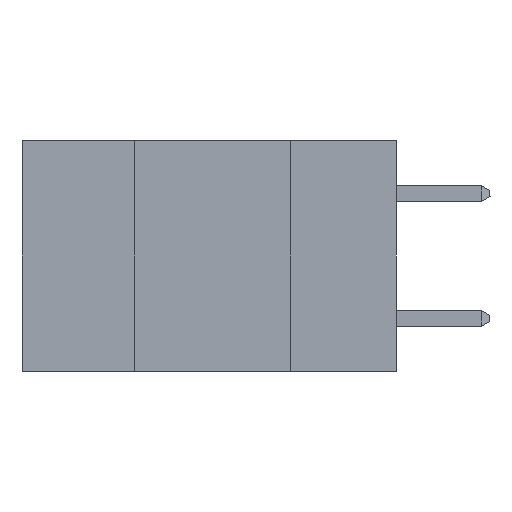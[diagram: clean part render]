
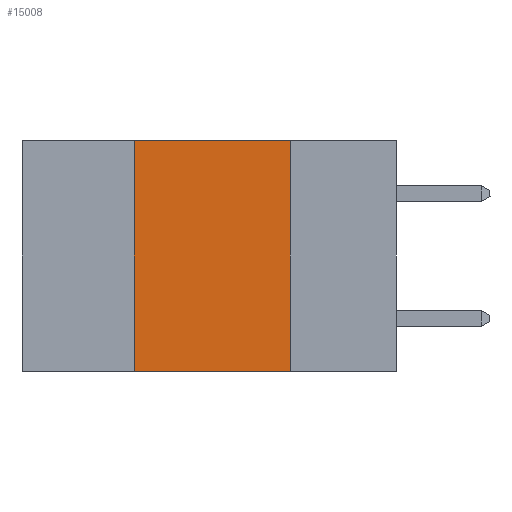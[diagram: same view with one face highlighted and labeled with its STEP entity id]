
A CAD part, left-side view. The second image highlights one B-rep face of the part: STEP entity #15008.
In plain terms, the highlighted planar face has unit normal (-1, 0, 0).
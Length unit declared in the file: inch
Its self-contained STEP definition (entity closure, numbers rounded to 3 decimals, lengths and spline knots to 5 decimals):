
#212 = EDGE_CURVE ( 'NONE', #6444, #10614, #8181, .T. ) ;
#1032 = FACE_OUTER_BOUND ( 'NONE', #9208, .T. ) ;
#1127 = CARTESIAN_POINT ( 'NONE',  ( 0., 0.42, 0. ) ) ;
#1214 = LINE ( 'NONE', #11741, #7696 ) ;
#1249 = VECTOR ( 'NONE', #15882, 39.37008 ) ;
#1621 = CARTESIAN_POINT ( 'NONE',  ( 0., 0.42, 0. ) ) ;
#1800 = VECTOR ( 'NONE', #9566, 39.37008 ) ;
#2646 = DIRECTION ( 'NONE',  ( 1., 0., 0. ) ) ;
#3077 = EDGE_CURVE ( 'NONE', #6444, #17207, #4253, .T. ) ;
#4253 = LINE ( 'NONE', #5194, #1800 ) ;
#4759 = CARTESIAN_POINT ( 'NONE',  ( 0., 0.17, 0. ) ) ;
#5026 = ORIENTED_EDGE ( 'NONE', *, *, #17885, .F. ) ;
#5194 = CARTESIAN_POINT ( 'NONE',  ( 0., 0.6, -0.37 ) ) ;
#5376 = ORIENTED_EDGE ( 'NONE', *, *, #6539, .F. ) ;
#6444 = VERTEX_POINT ( 'NONE', #7243 ) ;
#6539 = EDGE_CURVE ( 'NONE', #14490, #17207, #9212, .T. ) ;
#7243 = CARTESIAN_POINT ( 'NONE',  ( 0., 0.42, -0.37 ) ) ;
#7254 = DIRECTION ( 'NONE',  ( 0., -1., 0. ) ) ;
#7696 = VECTOR ( 'NONE', #7254, 39.37008 ) ;
#8181 = LINE ( 'NONE', #1621, #1249 ) ;
#8528 = VECTOR ( 'NONE', #16338, 39.37008 ) ;
#8595 = PLANE ( 'NONE',  #16510 ) ;
#9208 = EDGE_LOOP ( 'NONE', ( #5376, #5026, #14899, #17398 ) ) ;
#9212 = LINE ( 'NONE', #4759, #8528 ) ;
#9566 = DIRECTION ( 'NONE',  ( 0., -1., 0. ) ) ;
#10614 = VERTEX_POINT ( 'NONE', #1127 ) ;
#11391 = CARTESIAN_POINT ( 'NONE',  ( 0., 0.6, 0. ) ) ;
#11741 = CARTESIAN_POINT ( 'NONE',  ( 0., 0.6, 0. ) ) ;
#14043 = CARTESIAN_POINT ( 'NONE',  ( 0., 0.17, 0. ) ) ;
#14490 = VERTEX_POINT ( 'NONE', #14043 ) ;
#14899 = ORIENTED_EDGE ( 'NONE', *, *, #212, .F. ) ;
#15008 = ADVANCED_FACE ( 'NONE', ( #1032 ), #8595, .F. ) ;
#15882 = DIRECTION ( 'NONE',  ( 0., 0., 1. ) ) ;
#16338 = DIRECTION ( 'NONE',  ( 0., 0., -1. ) ) ;
#16510 = AXIS2_PLACEMENT_3D ( 'NONE', #11391, #2646, #18401 ) ;
#17064 = CARTESIAN_POINT ( 'NONE',  ( 0., 0.17, -0.37 ) ) ;
#17207 = VERTEX_POINT ( 'NONE', #17064 ) ;
#17398 = ORIENTED_EDGE ( 'NONE', *, *, #3077, .T. ) ;
#17885 = EDGE_CURVE ( 'NONE', #10614, #14490, #1214, .T. ) ;
#18401 = DIRECTION ( 'NONE',  ( 0., 0., -1. ) ) ;
